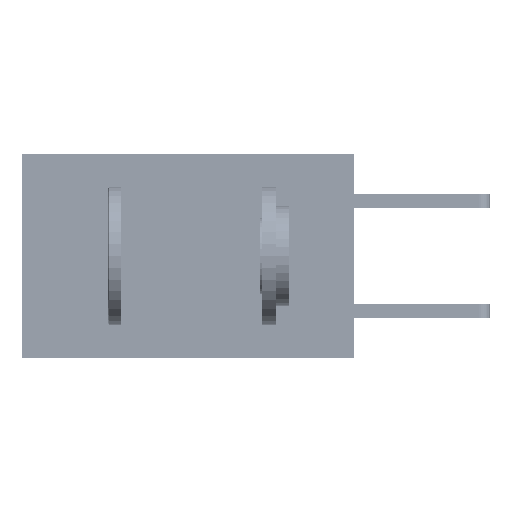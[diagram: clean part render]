
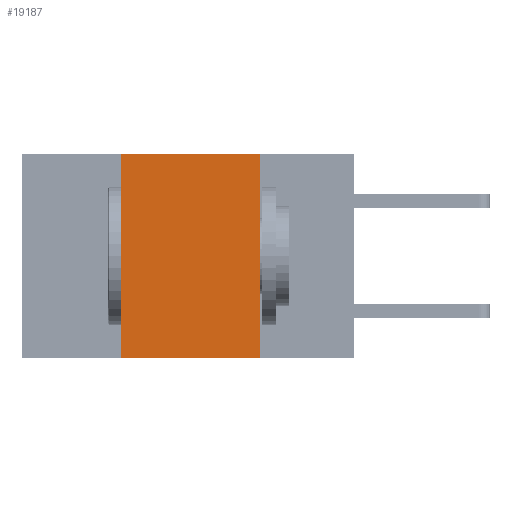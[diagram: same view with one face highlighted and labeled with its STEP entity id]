
A CAD part, left-side view. The second image highlights one B-rep face of the part: STEP entity #19187.
In plain terms, the highlighted planar face has unit normal (-1, 0, 0).
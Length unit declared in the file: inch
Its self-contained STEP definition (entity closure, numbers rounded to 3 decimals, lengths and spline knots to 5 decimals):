
#528 = LINE ( 'NONE', #35276, #8130 ) ;
#962 = EDGE_CURVE ( 'NONE', #31589, #26383, #528, .T. ) ;
#4630 = ORIENTED_EDGE ( 'NONE', *, *, #6430, .F. ) ;
#5179 = CARTESIAN_POINT ( 'NONE',  ( 0., 0.6, 0. ) ) ;
#6430 = EDGE_CURVE ( 'NONE', #26383, #37359, #32943, .T. ) ;
#6777 = VECTOR ( 'NONE', #14818, 39.37008 ) ;
#7208 = CARTESIAN_POINT ( 'NONE',  ( 0., 0.17, 0. ) ) ;
#8130 = VECTOR ( 'NONE', #29752, 39.37008 ) ;
#8133 = LINE ( 'NONE', #17453, #8632 ) ;
#8461 = VECTOR ( 'NONE', #32960, 39.37008 ) ;
#8632 = VECTOR ( 'NONE', #21629, 39.37008 ) ;
#10078 = EDGE_CURVE ( 'NONE', #36169, #31589, #8133, .T. ) ;
#10458 = FACE_OUTER_BOUND ( 'NONE', #32280, .T. ) ;
#11343 = AXIS2_PLACEMENT_3D ( 'NONE', #5179, #27559, #33259 ) ;
#11348 = ORIENTED_EDGE ( 'NONE', *, *, #962, .F. ) ;
#12799 = CARTESIAN_POINT ( 'NONE',  ( 0., 0.42, -0.37 ) ) ;
#14063 = ORIENTED_EDGE ( 'NONE', *, *, #35354, .T. ) ;
#14818 = DIRECTION ( 'NONE',  ( 0., -1., 0. ) ) ;
#17453 = CARTESIAN_POINT ( 'NONE',  ( 0., 0.42, 0. ) ) ;
#19187 = ADVANCED_FACE ( 'NONE', ( #10458 ), #24321, .F. ) ;
#19299 = CARTESIAN_POINT ( 'NONE',  ( 0., 0.17, 0. ) ) ;
#21629 = DIRECTION ( 'NONE',  ( 0., 0., 1. ) ) ;
#23809 = LINE ( 'NONE', #29988, #6777 ) ;
#24321 = PLANE ( 'NONE',  #11343 ) ;
#26382 = ORIENTED_EDGE ( 'NONE', *, *, #10078, .F. ) ;
#26383 = VERTEX_POINT ( 'NONE', #19299 ) ;
#27559 = DIRECTION ( 'NONE',  ( 1., 0., 0. ) ) ;
#29752 = DIRECTION ( 'NONE',  ( 0., -1., 0. ) ) ;
#29988 = CARTESIAN_POINT ( 'NONE',  ( 0., 0.6, -0.37 ) ) ;
#31589 = VERTEX_POINT ( 'NONE', #41433 ) ;
#32280 = EDGE_LOOP ( 'NONE', ( #4630, #11348, #26382, #14063 ) ) ;
#32943 = LINE ( 'NONE', #7208, #8461 ) ;
#32960 = DIRECTION ( 'NONE',  ( 0., 0., -1. ) ) ;
#33259 = DIRECTION ( 'NONE',  ( 0., 0., -1. ) ) ;
#35276 = CARTESIAN_POINT ( 'NONE',  ( 0., 0.6, 0. ) ) ;
#35354 = EDGE_CURVE ( 'NONE', #36169, #37359, #23809, .T. ) ;
#36169 = VERTEX_POINT ( 'NONE', #12799 ) ;
#37085 = CARTESIAN_POINT ( 'NONE',  ( 0., 0.17, -0.37 ) ) ;
#37359 = VERTEX_POINT ( 'NONE', #37085 ) ;
#41433 = CARTESIAN_POINT ( 'NONE',  ( 0., 0.42, 0. ) ) ;
